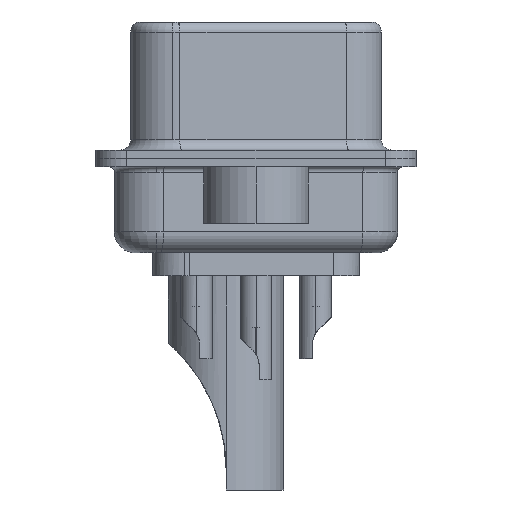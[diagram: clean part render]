
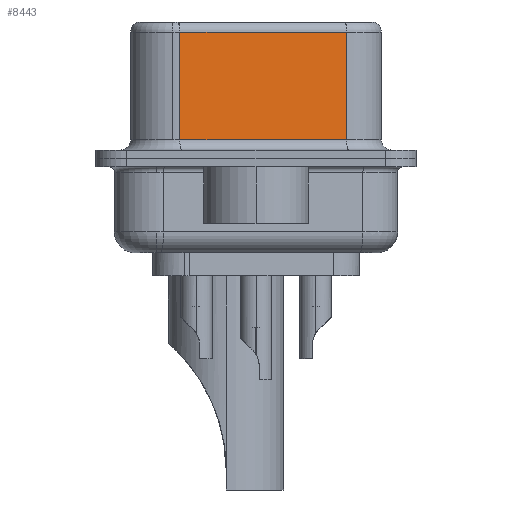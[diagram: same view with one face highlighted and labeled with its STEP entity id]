
A CAD part, left-side view. The second image highlights one B-rep face of the part: STEP entity #8443.
In plain terms, the highlighted planar face has unit normal (-0.985, -0.174, 0).
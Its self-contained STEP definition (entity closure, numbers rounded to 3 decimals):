
#305 = LINE ( 'NONE', #24807, #23257 ) ;
#496 = VERTEX_POINT ( 'NONE', #2898 ) ;
#2149 = AXIS2_PLACEMENT_3D ( 'NONE', #3273, #5573, #21069 ) ;
#2898 = CARTESIAN_POINT ( 'NONE',  ( 5.132, -4.322, 0.9 ) ) ;
#3088 = VERTEX_POINT ( 'NONE', #28677 ) ;
#3273 = CARTESIAN_POINT ( 'NONE',  ( 5.132, -4.322, 6.52 ) ) ;
#3696 = VERTEX_POINT ( 'NONE', #15223 ) ;
#3714 = ORIENTED_EDGE ( 'NONE', *, *, #10181, .T. ) ;
#5573 = DIRECTION ( 'NONE',  ( 0.985, 0.174, 0. ) ) ;
#8271 = VECTOR ( 'NONE', #12377, 1000. ) ;
#8443 = ADVANCED_FACE ( 'NONE', ( #14897 ), #16621, .F. ) ;
#10181 = EDGE_CURVE ( 'NONE', #3696, #3088, #26733, .T. ) ;
#11894 = CARTESIAN_POINT ( 'NONE',  ( 5.132, -4.322, 6.02 ) ) ;
#12327 = CARTESIAN_POINT ( 'NONE',  ( 5.132, -4.322, 6.52 ) ) ;
#12377 = DIRECTION ( 'NONE',  ( 0.174, -0.985, 0. ) ) ;
#12810 = EDGE_LOOP ( 'NONE', ( #18694, #3714, #23177, #16232 ) ) ;
#13056 = VECTOR ( 'NONE', #16183, 1000. ) ;
#13071 = LINE ( 'NONE', #12327, #24702 ) ;
#14897 = FACE_OUTER_BOUND ( 'NONE', #12810, .T. ) ;
#15223 = CARTESIAN_POINT ( 'NONE',  ( 5.132, -4.322, 6.02 ) ) ;
#16183 = DIRECTION ( 'NONE',  ( -0.174, 0.985, 0. ) ) ;
#16232 = ORIENTED_EDGE ( 'NONE', *, *, #25202, .T. ) ;
#16621 = PLANE ( 'NONE',  #2149 ) ;
#16764 = CARTESIAN_POINT ( 'NONE',  ( 5.132, -4.322, 0.9 ) ) ;
#18694 = ORIENTED_EDGE ( 'NONE', *, *, #28660, .F. ) ;
#19908 = EDGE_CURVE ( 'NONE', #3088, #23220, #305, .T. ) ;
#20687 = LINE ( 'NONE', #16764, #8271 ) ;
#21069 = DIRECTION ( 'NONE',  ( -0.174, 0.985, 0. ) ) ;
#21204 = CARTESIAN_POINT ( 'NONE',  ( 3.73, 3.628, 0.9 ) ) ;
#23177 = ORIENTED_EDGE ( 'NONE', *, *, #19908, .T. ) ;
#23220 = VERTEX_POINT ( 'NONE', #21204 ) ;
#23257 = VECTOR ( 'NONE', #26978, 1000. ) ;
#24702 = VECTOR ( 'NONE', #27591, 1000. ) ;
#24807 = CARTESIAN_POINT ( 'NONE',  ( 3.73, 3.628, 6.52 ) ) ;
#25202 = EDGE_CURVE ( 'NONE', #23220, #496, #20687, .T. ) ;
#26733 = LINE ( 'NONE', #11894, #13056 ) ;
#26978 = DIRECTION ( 'NONE',  ( 0., 0., -1. ) ) ;
#27591 = DIRECTION ( 'NONE',  ( 0., 0., -1. ) ) ;
#28660 = EDGE_CURVE ( 'NONE', #3696, #496, #13071, .T. ) ;
#28677 = CARTESIAN_POINT ( 'NONE',  ( 3.73, 3.628, 6.02 ) ) ;
